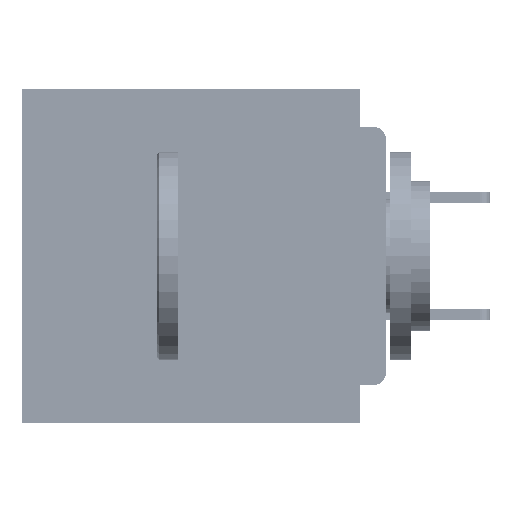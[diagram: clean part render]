
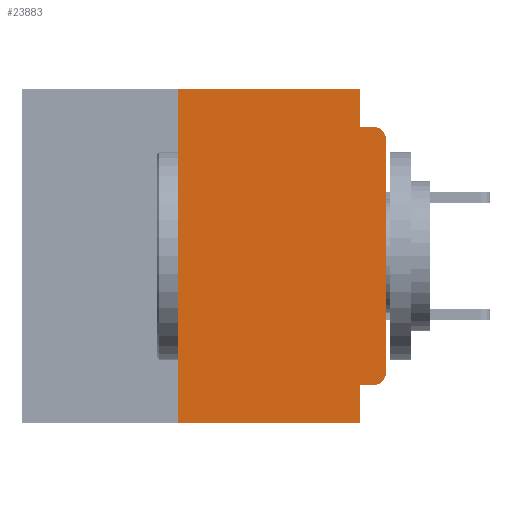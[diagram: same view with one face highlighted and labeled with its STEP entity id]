
A CAD part, left-side view. The second image highlights one B-rep face of the part: STEP entity #23883.
In plain terms, the highlighted planar face has unit normal (-1, 0, 0).
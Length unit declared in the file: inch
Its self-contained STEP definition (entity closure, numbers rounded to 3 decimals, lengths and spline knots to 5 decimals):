
#181 = EDGE_CURVE ( 'NONE', #26623, #33048, #46755, .T. ) ;
#2433 = LINE ( 'NONE', #43842, #13096 ) ;
#4372 = DIRECTION ( 'NONE',  ( 0., -1., 0. ) ) ;
#4424 = CARTESIAN_POINT ( 'NONE',  ( 0., 0., -0.355 ) ) ;
#6531 = ORIENTED_EDGE ( 'NONE', *, *, #15590, .T. ) ;
#7367 = CARTESIAN_POINT ( 'NONE',  ( 0., 0.031, -0.355 ) ) ;
#8191 = ORIENTED_EDGE ( 'NONE', *, *, #59775, .F. ) ;
#8463 = EDGE_CURVE ( 'NONE', #17199, #33048, #40198, .T. ) ;
#9664 = LINE ( 'NONE', #67277, #63875 ) ;
#12388 = CARTESIAN_POINT ( 'NONE',  ( 0., 0.015, -0.34 ) ) ;
#13096 = VECTOR ( 'NONE', #22969, 39.37008 ) ;
#13548 = VERTEX_POINT ( 'NONE', #62011 ) ;
#15590 = EDGE_CURVE ( 'NONE', #37751, #30843, #44317, .T. ) ;
#15595 = EDGE_CURVE ( 'NONE', #23418, #40272, #2433, .T. ) ;
#16196 = ORIENTED_EDGE ( 'NONE', *, *, #181, .T. ) ;
#17199 = VERTEX_POINT ( 'NONE', #28397 ) ;
#17639 = DIRECTION ( 'NONE',  ( 0., 0., -1. ) ) ;
#19104 = CARTESIAN_POINT ( 'NONE',  ( 0., 0., -0.34 ) ) ;
#19395 = AXIS2_PLACEMENT_3D ( 'NONE', #40366, #39827, #39906 ) ;
#20325 = EDGE_CURVE ( 'NONE', #30843, #26623, #62597, .T. ) ;
#21230 = CARTESIAN_POINT ( 'NONE',  ( 0., 0.031, -0.4 ) ) ;
#22969 = DIRECTION ( 'NONE',  ( 0., -1., 0. ) ) ;
#23347 = DIRECTION ( 'NONE',  ( 0., 0., 1. ) ) ;
#23418 = VERTEX_POINT ( 'NONE', #27335 ) ;
#23883 = ADVANCED_FACE ( 'NONE', ( #50465 ), #57597, .F. ) ;
#26126 = CARTESIAN_POINT ( 'NONE',  ( 0., 0.437, 0. ) ) ;
#26623 = VERTEX_POINT ( 'NONE', #33417 ) ;
#27175 = DIRECTION ( 'NONE',  ( 0., 0., 1. ) ) ;
#27335 = CARTESIAN_POINT ( 'NONE',  ( 0., 0.25, 0. ) ) ;
#27336 = CARTESIAN_POINT ( 'NONE',  ( 0., 0.015, -0.045 ) ) ;
#28397 = CARTESIAN_POINT ( 'NONE',  ( 0., 0.031, -0.045 ) ) ;
#29706 = EDGE_CURVE ( 'NONE', #37751, #48601, #43124, .T. ) ;
#30145 = CARTESIAN_POINT ( 'NONE',  ( 0., 0., -0.045 ) ) ;
#30843 = VERTEX_POINT ( 'NONE', #19104 ) ;
#31412 = DIRECTION ( 'NONE',  ( 1., 0., 0. ) ) ;
#32392 = EDGE_LOOP ( 'NONE', ( #32961, #16196, #60859, #61221, #55182, #8191, #68005, #63822, #56485, #6531 ) ) ;
#32961 = ORIENTED_EDGE ( 'NONE', *, *, #20325, .T. ) ;
#33048 = VERTEX_POINT ( 'NONE', #27336 ) ;
#33417 = CARTESIAN_POINT ( 'NONE',  ( 0., 0., -0.06 ) ) ;
#33832 = EDGE_CURVE ( 'NONE', #40272, #17199, #60574, .T. ) ;
#35570 = CARTESIAN_POINT ( 'NONE',  ( 0., 0.031, 0. ) ) ;
#36432 = CARTESIAN_POINT ( 'NONE',  ( 0., 0.031, 0. ) ) ;
#37751 = VERTEX_POINT ( 'NONE', #49874 ) ;
#38934 = CARTESIAN_POINT ( 'NONE',  ( 0., 0.25, -0.4 ) ) ;
#38985 = AXIS2_PLACEMENT_3D ( 'NONE', #26126, #31412, #54488 ) ;
#39154 = VERTEX_POINT ( 'NONE', #45333 ) ;
#39827 = DIRECTION ( 'NONE',  ( -1., 0., 0. ) ) ;
#39906 = DIRECTION ( 'NONE',  ( 0., 0., -1. ) ) ;
#40198 = LINE ( 'NONE', #30145, #66467 ) ;
#40272 = VERTEX_POINT ( 'NONE', #35570 ) ;
#40366 = CARTESIAN_POINT ( 'NONE',  ( 0., 0.015, -0.06 ) ) ;
#42544 = EDGE_CURVE ( 'NONE', #13548, #39154, #9664, .T. ) ;
#43124 = LINE ( 'NONE', #4424, #52195 ) ;
#43842 = CARTESIAN_POINT ( 'NONE',  ( 0., 0.437, 0. ) ) ;
#43873 = EDGE_CURVE ( 'NONE', #48601, #39154, #62058, .T. ) ;
#44317 = CIRCLE ( 'NONE', #46340, 0.015 ) ;
#45333 = CARTESIAN_POINT ( 'NONE',  ( 0., 0.031, -0.4 ) ) ;
#45565 = VECTOR ( 'NONE', #23347, 39.37008 ) ;
#46340 = AXIS2_PLACEMENT_3D ( 'NONE', #12388, #49130, #17639 ) ;
#46462 = VECTOR ( 'NONE', #52688, 39.37008 ) ;
#46477 = DIRECTION ( 'NONE',  ( 0., 1., 0. ) ) ;
#46600 = VECTOR ( 'NONE', #57581, 39.37008 ) ;
#46755 = CIRCLE ( 'NONE', #19395, 0.015 ) ;
#48601 = VERTEX_POINT ( 'NONE', #7367 ) ;
#49130 = DIRECTION ( 'NONE',  ( -1., 0., 0. ) ) ;
#49874 = CARTESIAN_POINT ( 'NONE',  ( 0., 0.015, -0.355 ) ) ;
#50465 = FACE_OUTER_BOUND ( 'NONE', #32392, .T. ) ;
#52195 = VECTOR ( 'NONE', #46477, 39.37008 ) ;
#52688 = DIRECTION ( 'NONE',  ( 0., 0., -1. ) ) ;
#54488 = DIRECTION ( 'NONE',  ( 0., 0., -1. ) ) ;
#55182 = ORIENTED_EDGE ( 'NONE', *, *, #15595, .F. ) ;
#56485 = ORIENTED_EDGE ( 'NONE', *, *, #29706, .F. ) ;
#57581 = DIRECTION ( 'NONE',  ( 0., 0., -1. ) ) ;
#57597 = PLANE ( 'NONE',  #38985 ) ;
#58620 = CARTESIAN_POINT ( 'NONE',  ( 0., 0., 0. ) ) ;
#59524 = LINE ( 'NONE', #38934, #45565 ) ;
#59775 = EDGE_CURVE ( 'NONE', #13548, #23418, #59524, .T. ) ;
#60574 = LINE ( 'NONE', #36432, #46600 ) ;
#60859 = ORIENTED_EDGE ( 'NONE', *, *, #8463, .F. ) ;
#60961 = VECTOR ( 'NONE', #27175, 39.37008 ) ;
#61221 = ORIENTED_EDGE ( 'NONE', *, *, #33832, .F. ) ;
#62011 = CARTESIAN_POINT ( 'NONE',  ( 0., 0.25, -0.4 ) ) ;
#62058 = LINE ( 'NONE', #21230, #46462 ) ;
#62597 = LINE ( 'NONE', #58620, #60961 ) ;
#63822 = ORIENTED_EDGE ( 'NONE', *, *, #43873, .F. ) ;
#63875 = VECTOR ( 'NONE', #4372, 39.37008 ) ;
#66467 = VECTOR ( 'NONE', #66846, 39.37008 ) ;
#66846 = DIRECTION ( 'NONE',  ( 0., -1., 0. ) ) ;
#67277 = CARTESIAN_POINT ( 'NONE',  ( 0., 0.437, -0.4 ) ) ;
#68005 = ORIENTED_EDGE ( 'NONE', *, *, #42544, .T. ) ;
